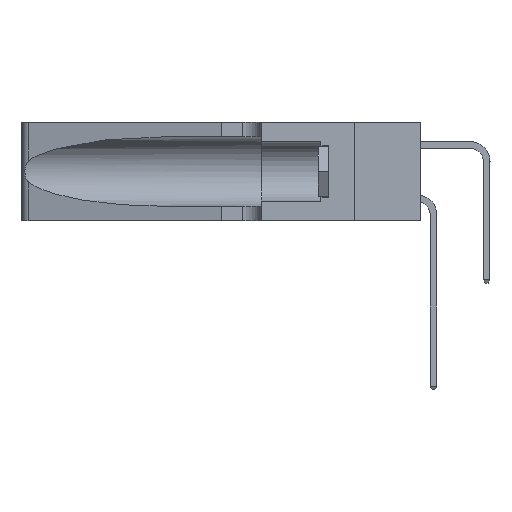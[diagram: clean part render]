
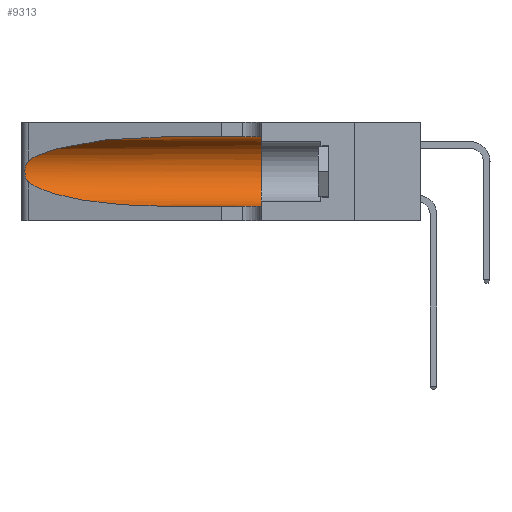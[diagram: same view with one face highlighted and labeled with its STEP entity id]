
A CAD part, left-side view. The second image highlights one B-rep face of the part: STEP entity #9313.
In plain terms, the highlighted cylindrical face has radius 3.308 mm (diameter 6.617 mm), a partial arc.
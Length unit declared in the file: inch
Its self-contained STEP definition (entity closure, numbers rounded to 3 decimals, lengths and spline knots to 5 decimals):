
#4 = CARTESIAN_POINT ( 'NONE',  ( 0.2373, 1.15595, 0.28018 ) ) ;
#192 = CARTESIAN_POINT ( 'NONE',  ( 0.25487, 1.22718, 0.22369 ) ) ;
#212 = AXIS2_PLACEMENT_3D ( 'NONE', #21553, #10229, #33009 ) ;
#802 =( BOUNDED_CURVE ( )  B_SPLINE_CURVE ( 3, ( #14849, #6428, #29271, #32125 ),
 .UNSPECIFIED., .F., .F. ) 
 B_SPLINE_CURVE_WITH_KNOTS ( ( 4, 4 ),
 ( 3.44316, 4.71239 ),
 .UNSPECIFIED. ) 
 CURVE ( )  GEOMETRIC_REPRESENTATION_ITEM ( )  RATIONAL_B_SPLINE_CURVE ( ( 1., 0.87, 0.87, 1. ) ) 
 REPRESENTATION_ITEM ( '' )  );
#1208 = CARTESIAN_POINT ( 'NONE',  ( 0.25789, 1.23486, 0.15765 ) ) ;
#1317 = VECTOR ( 'NONE', #28282, 39.37008 ) ;
#1334 = CARTESIAN_POINT ( 'NONE',  ( 0.25856, 1.23593, 0.16098 ) ) ;
#1466 = CARTESIAN_POINT ( 'NONE',  ( 0.25639, 1.23184, 0.21858 ) ) ;
#1667 = CARTESIAN_POINT ( 'NONE',  ( 0.1305, 0.35, 0.05475 ) ) ;
#3491 = CARTESIAN_POINT ( 'NONE',  ( 0.25487, 1.22718, 0.22369 ) ) ;
#3569 =( BOUNDED_CURVE ( )  B_SPLINE_CURVE ( 3, ( #16896, #20020, #4, #192 ),
 .UNSPECIFIED., .F., .F. ) 
 B_SPLINE_CURVE_WITH_KNOTS ( ( 4, 4 ),
 ( 1.5708, 2.84003 ),
 .UNSPECIFIED. ) 
 CURVE ( )  GEOMETRIC_REPRESENTATION_ITEM ( )  RATIONAL_B_SPLINE_CURVE ( ( 1., 0.87, 0.87, 1. ) ) 
 REPRESENTATION_ITEM ( '' )  );
#4096 = CARTESIAN_POINT ( 'NONE',  ( 0.25487, 1.22718, 0.14631 ) ) ;
#4985 = EDGE_LOOP ( 'NONE', ( #7258, #34212, #12429, #30816, #25599, #17781 ) ) ;
#5176 = CARTESIAN_POINT ( 'NONE',  ( 0.1305, 0.72297, 0.05475 ) ) ;
#5483 = EDGE_CURVE ( 'NONE', #12820, #35545, #8540, .T. ) ;
#6428 = CARTESIAN_POINT ( 'NONE',  ( 0.2373, 1.15595, 0.08982 ) ) ;
#7097 = CARTESIAN_POINT ( 'NONE',  ( 0.25555, 1.22993, 0.14849 ) ) ;
#7258 = ORIENTED_EDGE ( 'NONE', *, *, #31173, .T. ) ;
#7494 = VERTEX_POINT ( 'NONE', #15941 ) ;
#8540 = LINE ( 'NONE', #25583, #1317 ) ;
#9313 = ADVANCED_FACE ( 'NONE', ( #30931 ), #35837, .F. ) ;
#9417 = DIRECTION ( 'NONE',  ( 0., 1., 0. ) ) ;
#10200 = EDGE_CURVE ( 'NONE', #31867, #7494, #29960, .T. ) ;
#10229 = DIRECTION ( 'NONE',  ( 0., -1., 0. ) ) ;
#11256 = CARTESIAN_POINT ( 'NONE',  ( 0.25487, 1.22718, 0.14631 ) ) ;
#12192 = CIRCLE ( 'NONE', #14818, 0.13025 ) ;
#12429 = ORIENTED_EDGE ( 'NONE', *, *, #23686, .T. ) ;
#12820 = VERTEX_POINT ( 'NONE', #5176 ) ;
#13292 = CARTESIAN_POINT ( 'NONE',  ( 0.1305, 1.61858, 0.31525 ) ) ;
#14612 = CARTESIAN_POINT ( 'NONE',  ( 0.1305, 0.72297, 0.31525 ) ) ;
#14818 = AXIS2_PLACEMENT_3D ( 'NONE', #26252, #9417, #20632 ) ;
#14849 = CARTESIAN_POINT ( 'NONE',  ( 0.25487, 1.22718, 0.14631 ) ) ;
#15628 = VERTEX_POINT ( 'NONE', #11256 ) ;
#15941 = CARTESIAN_POINT ( 'NONE',  ( 0.1305, 0.35, 0.31525 ) ) ;
#16221 = DIRECTION ( 'NONE',  ( 0., -1., 0. ) ) ;
#16582 = VERTEX_POINT ( 'NONE', #27899 ) ;
#16896 = CARTESIAN_POINT ( 'NONE',  ( 0.1305, 0.72297, 0.31525 ) ) ;
#17494 = EDGE_CURVE ( 'NONE', #7494, #35545, #12192, .T. ) ;
#17781 = ORIENTED_EDGE ( 'NONE', *, *, #10200, .F. ) ;
#18269 = CARTESIAN_POINT ( 'NONE',  ( 0.26075, 1.23896, 0.19203 ) ) ;
#18649 = CARTESIAN_POINT ( 'NONE',  ( 0.26017, 1.23833, 0.17102 ) ) ;
#20020 = CARTESIAN_POINT ( 'NONE',  ( 0.18966, 0.96281, 0.31525 ) ) ;
#20632 = DIRECTION ( 'NONE',  ( 0., 0., 1. ) ) ;
#21553 = CARTESIAN_POINT ( 'NONE',  ( 0.1305, 1.61858, 0.185 ) ) ;
#21659 = CARTESIAN_POINT ( 'NONE',  ( 0.25639, 1.23186, 0.15144 ) ) ;
#21990 = VECTOR ( 'NONE', #16221, 39.37008 ) ;
#23686 = EDGE_CURVE ( 'NONE', #15628, #12820, #802, .T. ) ;
#24264 = CARTESIAN_POINT ( 'NONE',  ( 0.26075, 1.23896, 0.178 ) ) ;
#25583 = CARTESIAN_POINT ( 'NONE',  ( 0.1305, 1.61858, 0.05475 ) ) ;
#25599 = ORIENTED_EDGE ( 'NONE', *, *, #17494, .F. ) ;
#26252 = CARTESIAN_POINT ( 'NONE',  ( 0.1305, 0.35, 0.185 ) ) ;
#26755 = CARTESIAN_POINT ( 'NONE',  ( 0.25854, 1.2359, 0.20912 ) ) ;
#27899 = CARTESIAN_POINT ( 'NONE',  ( 0.25487, 1.22718, 0.22369 ) ) ;
#28282 = DIRECTION ( 'NONE',  ( 0., -1., 0. ) ) ;
#29271 = CARTESIAN_POINT ( 'NONE',  ( 0.18966, 0.96281, 0.05475 ) ) ;
#29331 = B_SPLINE_CURVE_WITH_KNOTS ( 'NONE', 3,
 ( #3491, #35818, #1466, #32977, #26755, #35439, #18269, #24264, #18649, #1334, #1208, #21659, #7097, #4096 ),
 .UNSPECIFIED., .F., .F.,
 ( 4, 2, 2, 2, 2, 2, 4 ),
 ( 0., 0.00027, 0.00053, 0.00107, 0.0016, 0.00187, 0.00214 ),
 .UNSPECIFIED. ) ;
#29960 = LINE ( 'NONE', #13292, #21990 ) ;
#30816 = ORIENTED_EDGE ( 'NONE', *, *, #5483, .T. ) ;
#30931 = FACE_OUTER_BOUND ( 'NONE', #4985, .T. ) ;
#31173 = EDGE_CURVE ( 'NONE', #31867, #16582, #3569, .T. ) ;
#31867 = VERTEX_POINT ( 'NONE', #14612 ) ;
#32125 = CARTESIAN_POINT ( 'NONE',  ( 0.1305, 0.72297, 0.05475 ) ) ;
#32655 = EDGE_CURVE ( 'NONE', #16582, #15628, #29331, .T. ) ;
#32977 = CARTESIAN_POINT ( 'NONE',  ( 0.25787, 1.23484, 0.2124 ) ) ;
#33009 = DIRECTION ( 'NONE',  ( 0., 0., -1. ) ) ;
#34212 = ORIENTED_EDGE ( 'NONE', *, *, #32655, .T. ) ;
#35439 = CARTESIAN_POINT ( 'NONE',  ( 0.26018, 1.23835, 0.19895 ) ) ;
#35545 = VERTEX_POINT ( 'NONE', #1667 ) ;
#35818 = CARTESIAN_POINT ( 'NONE',  ( 0.25555, 1.22994, 0.2215 ) ) ;
#35837 = CYLINDRICAL_SURFACE ( 'NONE', #212, 0.13025 ) ;
